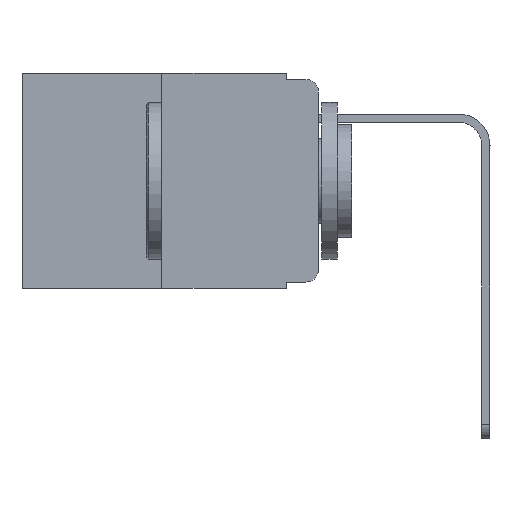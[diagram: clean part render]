
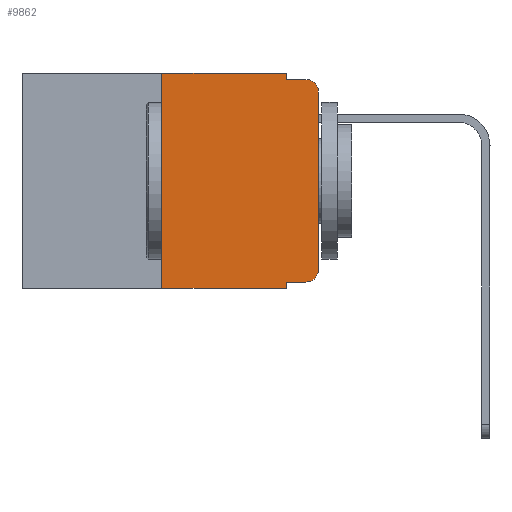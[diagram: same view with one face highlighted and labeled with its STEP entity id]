
A CAD part, left-side view. The second image highlights one B-rep face of the part: STEP entity #9862.
In plain terms, the highlighted planar face has unit normal (-1, 0, 0).
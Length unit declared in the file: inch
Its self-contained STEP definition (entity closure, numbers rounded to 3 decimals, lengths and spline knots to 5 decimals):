
#26 = VECTOR ( 'NONE', #4864, 39.37008 ) ;
#322 = VERTEX_POINT ( 'NONE', #9313 ) ;
#334 = LINE ( 'NONE', #10816, #12156 ) ;
#595 = ORIENTED_EDGE ( 'NONE', *, *, #1240, .T. ) ;
#738 = DIRECTION ( 'NONE',  ( 1., 0., 0. ) ) ;
#819 = VECTOR ( 'NONE', #12269, 39.37008 ) ;
#962 = CARTESIAN_POINT ( 'NONE',  ( 0., 0.25, 0. ) ) ;
#1240 = EDGE_CURVE ( 'NONE', #12037, #5206, #13080, .T. ) ;
#1342 = LINE ( 'NONE', #8388, #9309 ) ;
#1516 = CARTESIAN_POINT ( 'NONE',  ( 0., 0.051, 0. ) ) ;
#1554 = CARTESIAN_POINT ( 'NONE',  ( 0., 0.051, -0.343 ) ) ;
#1698 = ORIENTED_EDGE ( 'NONE', *, *, #13161, .F. ) ;
#1741 = VERTEX_POINT ( 'NONE', #962 ) ;
#1859 = CARTESIAN_POINT ( 'NONE',  ( 0., 0.473, 0. ) ) ;
#1998 = DIRECTION ( 'NONE',  ( 0., 0., -1. ) ) ;
#2011 = CARTESIAN_POINT ( 'NONE',  ( 0., 0., 0. ) ) ;
#2093 = ORIENTED_EDGE ( 'NONE', *, *, #3461, .F. ) ;
#2161 = FACE_OUTER_BOUND ( 'NONE', #12098, .T. ) ;
#2557 = LINE ( 'NONE', #7143, #10025 ) ;
#2703 = CARTESIAN_POINT ( 'NONE',  ( 0., 0., -0.313 ) ) ;
#2967 = ORIENTED_EDGE ( 'NONE', *, *, #13895, .T. ) ;
#3116 = DIRECTION ( 'NONE',  ( -1., 0., 0. ) ) ;
#3461 = EDGE_CURVE ( 'NONE', #4850, #1741, #334, .T. ) ;
#3593 = LINE ( 'NONE', #13386, #10020 ) ;
#4420 = VECTOR ( 'NONE', #13168, 39.37008 ) ;
#4442 = CARTESIAN_POINT ( 'NONE',  ( 0., 0.02, -0.01 ) ) ;
#4802 = ORIENTED_EDGE ( 'NONE', *, *, #8159, .T. ) ;
#4850 = VERTEX_POINT ( 'NONE', #9453 ) ;
#4864 = DIRECTION ( 'NONE',  ( 0., -1., 0. ) ) ;
#4936 = VERTEX_POINT ( 'NONE', #1554 ) ;
#4974 = ORIENTED_EDGE ( 'NONE', *, *, #9152, .T. ) ;
#5085 = AXIS2_PLACEMENT_3D ( 'NONE', #8691, #3116, #7484 ) ;
#5115 = EDGE_CURVE ( 'NONE', #4850, #4936, #7959, .T. ) ;
#5206 = VERTEX_POINT ( 'NONE', #5920 ) ;
#5568 = EDGE_CURVE ( 'NONE', #6243, #10991, #1342, .T. ) ;
#5888 = VERTEX_POINT ( 'NONE', #7593 ) ;
#5920 = CARTESIAN_POINT ( 'NONE',  ( 0., 0.02, -0.333 ) ) ;
#5983 = ORIENTED_EDGE ( 'NONE', *, *, #5568, .F. ) ;
#6086 = ORIENTED_EDGE ( 'NONE', *, *, #5115, .T. ) ;
#6243 = VERTEX_POINT ( 'NONE', #14184 ) ;
#6526 = DIRECTION ( 'NONE',  ( 0., 0., 1. ) ) ;
#7073 = CIRCLE ( 'NONE', #11329, 0.02 ) ;
#7100 = DIRECTION ( 'NONE',  ( 0., -1., 0. ) ) ;
#7143 = CARTESIAN_POINT ( 'NONE',  ( 0., 0.473, 0. ) ) ;
#7256 = DIRECTION ( 'NONE',  ( -1., 0., 0. ) ) ;
#7351 = DIRECTION ( 'NONE',  ( 0., 0., -1. ) ) ;
#7475 = CARTESIAN_POINT ( 'NONE',  ( 0., 0.051, -0.333 ) ) ;
#7484 = DIRECTION ( 'NONE',  ( 0., 0., -1. ) ) ;
#7593 = CARTESIAN_POINT ( 'NONE',  ( 0., 0.051, 0. ) ) ;
#7772 = ORIENTED_EDGE ( 'NONE', *, *, #12322, .F. ) ;
#7959 = LINE ( 'NONE', #12221, #819 ) ;
#8080 = DIRECTION ( 'NONE',  ( 0., 0., -1. ) ) ;
#8159 = EDGE_CURVE ( 'NONE', #12598, #322, #13663, .T. ) ;
#8388 = CARTESIAN_POINT ( 'NONE',  ( 0., 0.051, -0.01 ) ) ;
#8691 = CARTESIAN_POINT ( 'NONE',  ( 0., 0.02, -0.313 ) ) ;
#9052 = AXIS2_PLACEMENT_3D ( 'NONE', #1859, #738, #1998 ) ;
#9152 = EDGE_CURVE ( 'NONE', #322, #10991, #7073, .T. ) ;
#9309 = VECTOR ( 'NONE', #13128, 39.37008 ) ;
#9313 = CARTESIAN_POINT ( 'NONE',  ( 0., 0., -0.03 ) ) ;
#9453 = CARTESIAN_POINT ( 'NONE',  ( 0., 0.25, -0.343 ) ) ;
#9825 = CIRCLE ( 'NONE', #5085, 0.02 ) ;
#9862 = ADVANCED_FACE ( 'NONE', ( #2161 ), #10807, .F. ) ;
#10020 = VECTOR ( 'NONE', #12349, 39.37008 ) ;
#10025 = VECTOR ( 'NONE', #7100, 39.37008 ) ;
#10256 = EDGE_CURVE ( 'NONE', #5888, #6243, #13643, .T. ) ;
#10807 = PLANE ( 'NONE',  #9052 ) ;
#10816 = CARTESIAN_POINT ( 'NONE',  ( 0., 0.25, 0. ) ) ;
#10850 = VECTOR ( 'NONE', #8080, 39.37008 ) ;
#10991 = VERTEX_POINT ( 'NONE', #4442 ) ;
#11102 = ORIENTED_EDGE ( 'NONE', *, *, #10256, .F. ) ;
#11329 = AXIS2_PLACEMENT_3D ( 'NONE', #11700, #7256, #7351 ) ;
#11553 = CARTESIAN_POINT ( 'NONE',  ( 0., 0.051, -0.333 ) ) ;
#11700 = CARTESIAN_POINT ( 'NONE',  ( 0., 0.02, -0.03 ) ) ;
#12037 = VERTEX_POINT ( 'NONE', #7475 ) ;
#12098 = EDGE_LOOP ( 'NONE', ( #4802, #4974, #5983, #11102, #1698, #2093, #6086, #7772, #595, #2967 ) ) ;
#12156 = VECTOR ( 'NONE', #6526, 39.37008 ) ;
#12221 = CARTESIAN_POINT ( 'NONE',  ( 0., 0.473, -0.343 ) ) ;
#12269 = DIRECTION ( 'NONE',  ( 0., -1., 0. ) ) ;
#12322 = EDGE_CURVE ( 'NONE', #12037, #4936, #3593, .T. ) ;
#12349 = DIRECTION ( 'NONE',  ( 0., 0., -1. ) ) ;
#12598 = VERTEX_POINT ( 'NONE', #2703 ) ;
#13080 = LINE ( 'NONE', #11553, #26 ) ;
#13128 = DIRECTION ( 'NONE',  ( 0., -1., 0. ) ) ;
#13161 = EDGE_CURVE ( 'NONE', #1741, #5888, #2557, .T. ) ;
#13168 = DIRECTION ( 'NONE',  ( 0., 0., 1. ) ) ;
#13386 = CARTESIAN_POINT ( 'NONE',  ( 0., 0.051, 0. ) ) ;
#13643 = LINE ( 'NONE', #1516, #10850 ) ;
#13663 = LINE ( 'NONE', #2011, #4420 ) ;
#13895 = EDGE_CURVE ( 'NONE', #5206, #12598, #9825, .T. ) ;
#14184 = CARTESIAN_POINT ( 'NONE',  ( 0., 0.051, -0.01 ) ) ;
